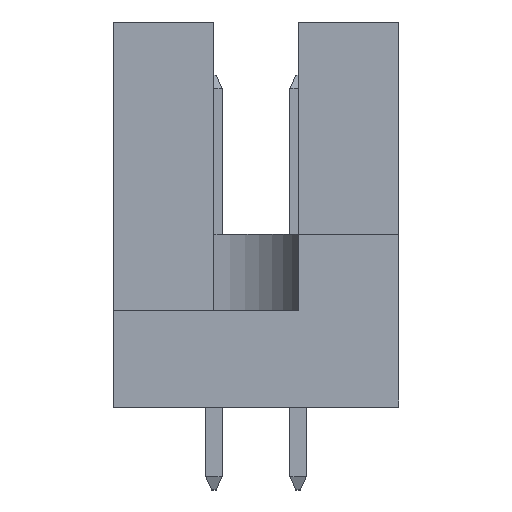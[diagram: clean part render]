
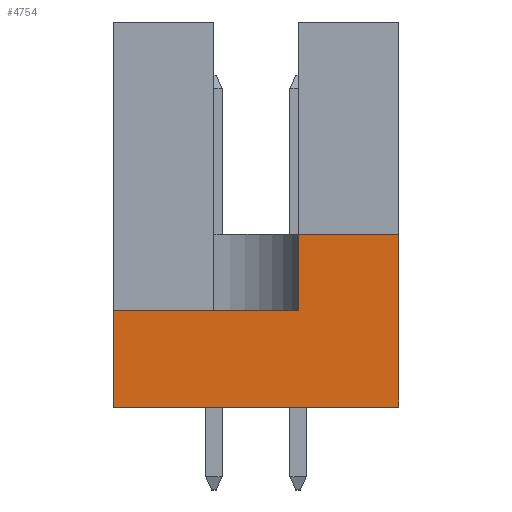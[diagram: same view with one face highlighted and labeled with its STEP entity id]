
A CAD part, left-side view. The second image highlights one B-rep face of the part: STEP entity #4754.
In plain terms, the highlighted planar face has unit normal (-1, 0, 0).
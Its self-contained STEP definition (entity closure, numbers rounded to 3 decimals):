
#245 = DIRECTION ( 'NONE',  ( 1., 0., 0. ) ) ;
#447 = DIRECTION ( 'NONE',  ( 0., 1., 0. ) ) ;
#616 = AXIS2_PLACEMENT_3D ( 'NONE', #4248, #245, #2550 ) ;
#743 = FACE_OUTER_BOUND ( 'NONE', #1087, .T. ) ;
#1087 = EDGE_LOOP ( 'NONE', ( #1671, #2449, #2115, #1414, #4751, #3703 ) ) ;
#1181 = CARTESIAN_POINT ( 'NONE',  ( -27.5, 4.3, 5.2 ) ) ;
#1407 = CARTESIAN_POINT ( 'NONE',  ( -27.5, -1.27, 5.2 ) ) ;
#1414 = ORIENTED_EDGE ( 'NONE', *, *, #2059, .T. ) ;
#1458 = VECTOR ( 'NONE', #6374, 1000. ) ;
#1565 = VERTEX_POINT ( 'NONE', #4461 ) ;
#1671 = ORIENTED_EDGE ( 'NONE', *, *, #3097, .F. ) ;
#2059 = EDGE_CURVE ( 'NONE', #1565, #3779, #4712, .T. ) ;
#2115 = ORIENTED_EDGE ( 'NONE', *, *, #2791, .T. ) ;
#2327 = CARTESIAN_POINT ( 'NONE',  ( -27.5, 4.3, 0. ) ) ;
#2449 = ORIENTED_EDGE ( 'NONE', *, *, #2910, .T. ) ;
#2550 = DIRECTION ( 'NONE',  ( 0., 0., -1. ) ) ;
#2646 = CARTESIAN_POINT ( 'NONE',  ( -27.5, 4.3, 0. ) ) ;
#2791 = EDGE_CURVE ( 'NONE', #5552, #1565, #7418, .T. ) ;
#2841 = CARTESIAN_POINT ( 'NONE',  ( -27.5, 4.3, 2.9 ) ) ;
#2910 = EDGE_CURVE ( 'NONE', #7241, #5552, #4998, .T. ) ;
#2972 = DIRECTION ( 'NONE',  ( 0., 0., -1. ) ) ;
#3097 = EDGE_CURVE ( 'NONE', #7241, #7292, #6359, .T. ) ;
#3195 = VERTEX_POINT ( 'NONE', #4307 ) ;
#3203 = VECTOR ( 'NONE', #6821, 1000. ) ;
#3648 = PLANE ( 'NONE',  #616 ) ;
#3703 = ORIENTED_EDGE ( 'NONE', *, *, #5380, .F. ) ;
#3779 = VERTEX_POINT ( 'NONE', #2646 ) ;
#3851 = CARTESIAN_POINT ( 'NONE',  ( -27.5, -4.3, 5.2 ) ) ;
#4248 = CARTESIAN_POINT ( 'NONE',  ( -27.5, 4.3, 11.6 ) ) ;
#4307 = CARTESIAN_POINT ( 'NONE',  ( -27.5, -4.3, 0. ) ) ;
#4442 = EDGE_CURVE ( 'NONE', #3779, #3195, #6944, .T. ) ;
#4461 = CARTESIAN_POINT ( 'NONE',  ( -27.5, 4.3, 2.9 ) ) ;
#4712 = LINE ( 'NONE', #6907, #6406 ) ;
#4733 = VECTOR ( 'NONE', #7054, 1000. ) ;
#4751 = ORIENTED_EDGE ( 'NONE', *, *, #4442, .T. ) ;
#4754 = ADVANCED_FACE ( 'NONE', ( #743 ), #3648, .F. ) ;
#4998 = LINE ( 'NONE', #6975, #4733 ) ;
#5299 = CARTESIAN_POINT ( 'NONE',  ( -27.5, -4.3, 11.6 ) ) ;
#5380 = EDGE_CURVE ( 'NONE', #7292, #3195, #5938, .T. ) ;
#5552 = VERTEX_POINT ( 'NONE', #6953 ) ;
#5938 = LINE ( 'NONE', #5299, #3203 ) ;
#6070 = VECTOR ( 'NONE', #7078, 1000. ) ;
#6359 = LINE ( 'NONE', #1181, #6070 ) ;
#6374 = DIRECTION ( 'NONE',  ( 0., -1., 0. ) ) ;
#6406 = VECTOR ( 'NONE', #2972, 1000. ) ;
#6413 = VECTOR ( 'NONE', #447, 1000. ) ;
#6821 = DIRECTION ( 'NONE',  ( 0., 0., -1. ) ) ;
#6907 = CARTESIAN_POINT ( 'NONE',  ( -27.5, 4.3, 11.6 ) ) ;
#6944 = LINE ( 'NONE', #2327, #1458 ) ;
#6953 = CARTESIAN_POINT ( 'NONE',  ( -27.5, -1.27, 2.9 ) ) ;
#6975 = CARTESIAN_POINT ( 'NONE',  ( -27.5, -1.27, 19.22 ) ) ;
#7054 = DIRECTION ( 'NONE',  ( 0., 0., -1. ) ) ;
#7078 = DIRECTION ( 'NONE',  ( 0., -1., 0. ) ) ;
#7241 = VERTEX_POINT ( 'NONE', #1407 ) ;
#7292 = VERTEX_POINT ( 'NONE', #3851 ) ;
#7418 = LINE ( 'NONE', #2841, #6413 ) ;
